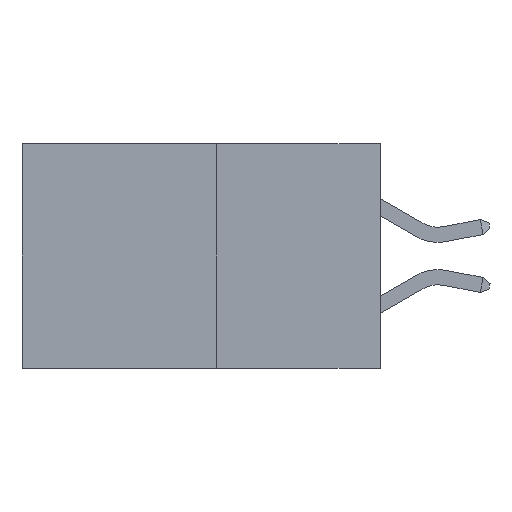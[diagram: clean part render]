
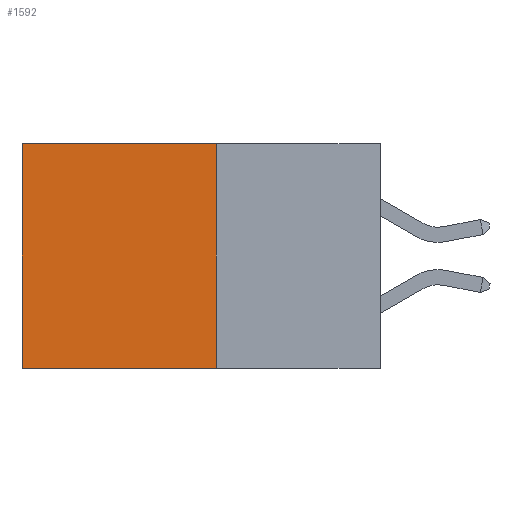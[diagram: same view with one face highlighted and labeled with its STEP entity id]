
A CAD part, left-side view. The second image highlights one B-rep face of the part: STEP entity #1592.
In plain terms, the highlighted planar face has unit normal (-1, 0, 0).
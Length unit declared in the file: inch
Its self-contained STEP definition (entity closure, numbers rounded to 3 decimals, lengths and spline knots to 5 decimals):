
#187 = DIRECTION ( 'NONE',  ( 1., 0., 0. ) ) ;
#242 = CARTESIAN_POINT ( 'NONE',  ( 0.277, 0.59, -0.37 ) ) ;
#673 = DIRECTION ( 'NONE',  ( 0., 0., -1. ) ) ;
#1592 = ADVANCED_FACE ( 'NONE', ( #8797 ), #6557, .F. ) ;
#1871 = VERTEX_POINT ( 'NONE', #16580 ) ;
#2063 = EDGE_CURVE ( 'NONE', #8523, #13688, #15003, .T. ) ;
#2624 = CARTESIAN_POINT ( 'NONE',  ( 0.277, 0.27, -0.37 ) ) ;
#2916 = EDGE_CURVE ( 'NONE', #7674, #1871, #18302, .T. ) ;
#4003 = VECTOR ( 'NONE', #11434, 39.37008 ) ;
#4135 = AXIS2_PLACEMENT_3D ( 'NONE', #6579, #187, #673 ) ;
#5027 = LINE ( 'NONE', #15559, #17213 ) ;
#5138 = VECTOR ( 'NONE', #14984, 39.37008 ) ;
#5644 = EDGE_CURVE ( 'NONE', #8523, #7674, #5027, .T. ) ;
#6115 = CARTESIAN_POINT ( 'NONE',  ( 0.277, 0.27, 0. ) ) ;
#6342 = CARTESIAN_POINT ( 'NONE',  ( 0.277, 0.27, 0. ) ) ;
#6543 = VECTOR ( 'NONE', #8800, 39.37008 ) ;
#6557 = PLANE ( 'NONE',  #4135 ) ;
#6579 = CARTESIAN_POINT ( 'NONE',  ( 0.277, 0.27, -0.37 ) ) ;
#7674 = VERTEX_POINT ( 'NONE', #16539 ) ;
#8523 = VERTEX_POINT ( 'NONE', #6342 ) ;
#8797 = FACE_OUTER_BOUND ( 'NONE', #16415, .T. ) ;
#8800 = DIRECTION ( 'NONE',  ( 0., 1., 0. ) ) ;
#9073 = CARTESIAN_POINT ( 'NONE',  ( 0.277, 0.59, 0. ) ) ;
#11434 = DIRECTION ( 'NONE',  ( 0., 0., -1. ) ) ;
#11487 = LINE ( 'NONE', #242, #4003 ) ;
#12644 = ORIENTED_EDGE ( 'NONE', *, *, #16215, .T. ) ;
#13688 = VERTEX_POINT ( 'NONE', #9073 ) ;
#14581 = DIRECTION ( 'NONE',  ( 0., 0., -1. ) ) ;
#14984 = DIRECTION ( 'NONE',  ( 0., 1., 0. ) ) ;
#15003 = LINE ( 'NONE', #6115, #6543 ) ;
#15120 = ORIENTED_EDGE ( 'NONE', *, *, #2916, .F. ) ;
#15559 = CARTESIAN_POINT ( 'NONE',  ( 0.277, 0.27, -0.37 ) ) ;
#16215 = EDGE_CURVE ( 'NONE', #13688, #1871, #11487, .T. ) ;
#16415 = EDGE_LOOP ( 'NONE', ( #12644, #15120, #19256, #20572 ) ) ;
#16539 = CARTESIAN_POINT ( 'NONE',  ( 0.277, 0.27, -0.37 ) ) ;
#16580 = CARTESIAN_POINT ( 'NONE',  ( 0.277, 0.59, -0.37 ) ) ;
#17213 = VECTOR ( 'NONE', #14581, 39.37008 ) ;
#18302 = LINE ( 'NONE', #2624, #5138 ) ;
#19256 = ORIENTED_EDGE ( 'NONE', *, *, #5644, .F. ) ;
#20572 = ORIENTED_EDGE ( 'NONE', *, *, #2063, .T. ) ;
